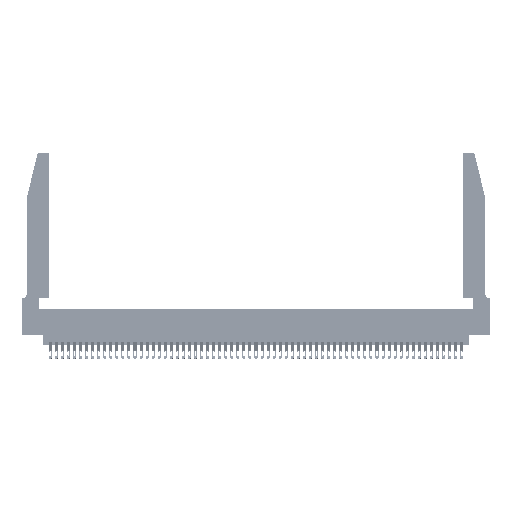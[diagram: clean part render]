
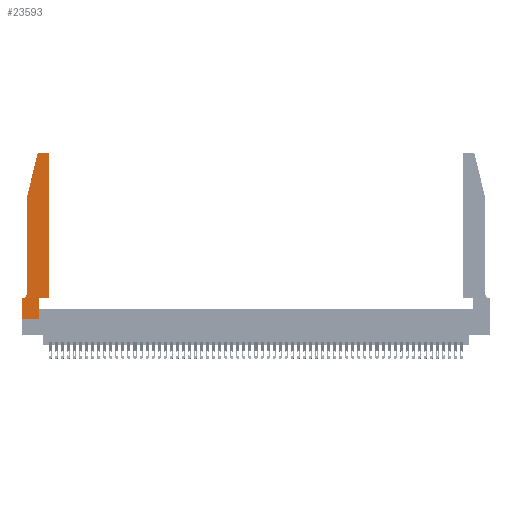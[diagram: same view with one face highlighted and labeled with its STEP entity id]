
A CAD part, top view. The second image highlights one B-rep face of the part: STEP entity #23593.
In plain terms, the highlighted planar face has unit normal (0, 0, 1).
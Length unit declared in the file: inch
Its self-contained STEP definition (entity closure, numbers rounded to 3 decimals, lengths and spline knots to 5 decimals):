
#453 = VERTEX_POINT ( 'NONE', #45107 ) ;
#953 = VECTOR ( 'NONE', #19039, 39.37008 ) ;
#2607 = VERTEX_POINT ( 'NONE', #25401 ) ;
#3213 = CARTESIAN_POINT ( 'NONE',  ( 0., 0., 0.37 ) ) ;
#3662 = DIRECTION ( 'NONE',  ( 1., 0., 0. ) ) ;
#3733 = EDGE_CURVE ( 'NONE', #24428, #12668, #29117, .T. ) ;
#5979 = DIRECTION ( 'NONE',  ( -0.239, -0.971, 0. ) ) ;
#7363 = ORIENTED_EDGE ( 'NONE', *, *, #15583, .T. ) ;
#8002 = EDGE_CURVE ( 'NONE', #31827, #35027, #25363, .T. ) ;
#8345 = DIRECTION ( 'NONE',  ( 1., 0., 0. ) ) ;
#8566 = ORIENTED_EDGE ( 'NONE', *, *, #44589, .T. ) ;
#9231 = CARTESIAN_POINT ( 'NONE',  ( 0.0755, 0.42, 0.37 ) ) ;
#10123 = LINE ( 'NONE', #43237, #31697 ) ;
#10504 = EDGE_CURVE ( 'NONE', #46183, #52420, #33589, .T. ) ;
#10516 = LINE ( 'NONE', #42050, #54915 ) ;
#11912 = DIRECTION ( 'NONE',  ( 0., 0., 1. ) ) ;
#12668 = VERTEX_POINT ( 'NONE', #22590 ) ;
#13037 = EDGE_CURVE ( 'NONE', #26854, #24428, #10516, .T. ) ;
#13666 = CARTESIAN_POINT ( 'NONE',  ( 0.2865, 0.35, 0.37 ) ) ;
#13884 = VECTOR ( 'NONE', #37668, 39.37008 ) ;
#14124 = CARTESIAN_POINT ( 'NONE',  ( 0.4505, 2.72, 0.37 ) ) ;
#14908 = VECTOR ( 'NONE', #5979, 39.37008 ) ;
#15583 = EDGE_CURVE ( 'NONE', #35027, #453, #30319, .T. ) ;
#15798 = EDGE_CURVE ( 'NONE', #453, #41656, #42335, .T. ) ;
#17495 = DIRECTION ( 'NONE',  ( 1., 0., 0. ) ) ;
#17571 = CIRCLE ( 'NONE', #42606, 0.03 ) ;
#17609 = ORIENTED_EDGE ( 'NONE', *, *, #31073, .T. ) ;
#17634 = EDGE_LOOP ( 'NONE', ( #17609, #20155, #27288, #55629, #39553, #28081, #48939, #7363, #45273, #8566, #20309, #40955 ) ) ;
#17738 = DIRECTION ( 'NONE',  ( 0., 0., -1. ) ) ;
#19039 = DIRECTION ( 'NONE',  ( -1., 0., 0. ) ) ;
#20155 = ORIENTED_EDGE ( 'NONE', *, *, #44213, .T. ) ;
#20309 = ORIENTED_EDGE ( 'NONE', *, *, #13037, .T. ) ;
#20850 = CARTESIAN_POINT ( 'NONE',  ( 0., 0., 0.37 ) ) ;
#22177 = VECTOR ( 'NONE', #41033, 39.37008 ) ;
#22448 = DIRECTION ( 'NONE',  ( 0., 0., 1. ) ) ;
#22590 = CARTESIAN_POINT ( 'NONE',  ( 0.4205, 2.75, 0.37 ) ) ;
#23593 = ADVANCED_FACE ( 'NONE', ( #33770 ), #29826, .T. ) ;
#24428 = VERTEX_POINT ( 'NONE', #14124 ) ;
#25363 = LINE ( 'NONE', #3213, #13884 ) ;
#25401 = CARTESIAN_POINT ( 'NONE',  ( 0.0055, 0.35, 0.37 ) ) ;
#26854 = VERTEX_POINT ( 'NONE', #39546 ) ;
#27288 = ORIENTED_EDGE ( 'NONE', *, *, #49001, .T. ) ;
#28081 = ORIENTED_EDGE ( 'NONE', *, *, #52580, .T. ) ;
#28804 = CARTESIAN_POINT ( 'NONE',  ( 0.0755, 2., 0.37 ) ) ;
#29117 = CIRCLE ( 'NONE', #54534, 0.03 ) ;
#29186 = CARTESIAN_POINT ( 'NONE',  ( 0.2865, 0.35, 0.37 ) ) ;
#29256 = VECTOR ( 'NONE', #31855, 39.37008 ) ;
#29483 = CARTESIAN_POINT ( 'NONE',  ( 0., 0.35, 0.37 ) ) ;
#29826 = PLANE ( 'NONE',  #43368 ) ;
#30319 = LINE ( 'NONE', #20850, #40374 ) ;
#30976 = VECTOR ( 'NONE', #43753, 39.37008 ) ;
#31073 = EDGE_CURVE ( 'NONE', #12668, #34992, #39328, .T. ) ;
#31697 = VECTOR ( 'NONE', #17495, 39.37008 ) ;
#31814 = CARTESIAN_POINT ( 'NONE',  ( 0.0755, 2., 0.37 ) ) ;
#31827 = VERTEX_POINT ( 'NONE', #29483 ) ;
#31855 = DIRECTION ( 'NONE',  ( -1., 0., 0. ) ) ;
#32761 = CARTESIAN_POINT ( 'NONE',  ( 0.0755, 2., 0.37 ) ) ;
#33589 = LINE ( 'NONE', #32761, #22177 ) ;
#33770 = FACE_OUTER_BOUND ( 'NONE', #17634, .T. ) ;
#34125 = DIRECTION ( 'NONE',  ( 0., 0., 1. ) ) ;
#34992 = VERTEX_POINT ( 'NONE', #38609 ) ;
#35013 = VERTEX_POINT ( 'NONE', #43098 ) ;
#35027 = VERTEX_POINT ( 'NONE', #51776 ) ;
#35319 = LINE ( 'NONE', #40456, #953 ) ;
#37668 = DIRECTION ( 'NONE',  ( 0., -1., 0. ) ) ;
#37674 = CARTESIAN_POINT ( 'NONE',  ( 0.4205, 2.72, 0.37 ) ) ;
#38609 = CARTESIAN_POINT ( 'NONE',  ( 0.284, 2.75, 0.37 ) ) ;
#39328 = LINE ( 'NONE', #40463, #29256 ) ;
#39546 = CARTESIAN_POINT ( 'NONE',  ( 0.4505, 0.35, 0.37 ) ) ;
#39553 = ORIENTED_EDGE ( 'NONE', *, *, #45771, .T. ) ;
#40374 = VECTOR ( 'NONE', #3662, 39.37008 ) ;
#40456 = CARTESIAN_POINT ( 'NONE',  ( 0.0755, 0.35, 0.37 ) ) ;
#40463 = CARTESIAN_POINT ( 'NONE',  ( 0.2605, 2.75, 0.37 ) ) ;
#40955 = ORIENTED_EDGE ( 'NONE', *, *, #3733, .T. ) ;
#41033 = DIRECTION ( 'NONE',  ( 0., -1., 0. ) ) ;
#41246 = AXIS2_PLACEMENT_3D ( 'NONE', #43471, #17738, #47817 ) ;
#41656 = VERTEX_POINT ( 'NONE', #29186 ) ;
#41992 = DIRECTION ( 'NONE',  ( 1., 0., 0. ) ) ;
#42050 = CARTESIAN_POINT ( 'NONE',  ( 0.4505, 0.35, 0.37 ) ) ;
#42335 = LINE ( 'NONE', #13666, #30976 ) ;
#42606 = AXIS2_PLACEMENT_3D ( 'NONE', #48177, #22448, #52530 ) ;
#43098 = CARTESIAN_POINT ( 'NONE',  ( 0.25487, 2.72718, 0.37 ) ) ;
#43237 = CARTESIAN_POINT ( 'NONE',  ( 0.4505, 0.35, 0.37 ) ) ;
#43368 = AXIS2_PLACEMENT_3D ( 'NONE', #51253, #34125, #8345 ) ;
#43471 = CARTESIAN_POINT ( 'NONE',  ( 0.0055, 0.42, 0.37 ) ) ;
#43753 = DIRECTION ( 'NONE',  ( 0., 1., 0. ) ) ;
#44213 = EDGE_CURVE ( 'NONE', #34992, #35013, #17571, .T. ) ;
#44589 = EDGE_CURVE ( 'NONE', #41656, #26854, #10123, .T. ) ;
#45107 = CARTESIAN_POINT ( 'NONE',  ( 0.2865, 0., 0.37 ) ) ;
#45273 = ORIENTED_EDGE ( 'NONE', *, *, #15798, .T. ) ;
#45771 = EDGE_CURVE ( 'NONE', #52420, #2607, #51019, .T. ) ;
#46183 = VERTEX_POINT ( 'NONE', #28804 ) ;
#47817 = DIRECTION ( 'NONE',  ( -1., 0., 0. ) ) ;
#48177 = CARTESIAN_POINT ( 'NONE',  ( 0.284, 2.72, 0.37 ) ) ;
#48939 = ORIENTED_EDGE ( 'NONE', *, *, #8002, .T. ) ;
#49001 = EDGE_CURVE ( 'NONE', #35013, #46183, #50557, .T. ) ;
#50557 = LINE ( 'NONE', #31814, #14908 ) ;
#51019 = CIRCLE ( 'NONE', #41246, 0.07 ) ;
#51253 = CARTESIAN_POINT ( 'NONE',  ( 0., 0.35, 0.37 ) ) ;
#51776 = CARTESIAN_POINT ( 'NONE',  ( 0., 0., 0.37 ) ) ;
#52420 = VERTEX_POINT ( 'NONE', #9231 ) ;
#52530 = DIRECTION ( 'NONE',  ( 1., 0., 0. ) ) ;
#52580 = EDGE_CURVE ( 'NONE', #2607, #31827, #35319, .T. ) ;
#54534 = AXIS2_PLACEMENT_3D ( 'NONE', #37674, #11912, #41992 ) ;
#54915 = VECTOR ( 'NONE', #55044, 39.37008 ) ;
#55044 = DIRECTION ( 'NONE',  ( 0., 1., 0. ) ) ;
#55629 = ORIENTED_EDGE ( 'NONE', *, *, #10504, .T. ) ;
